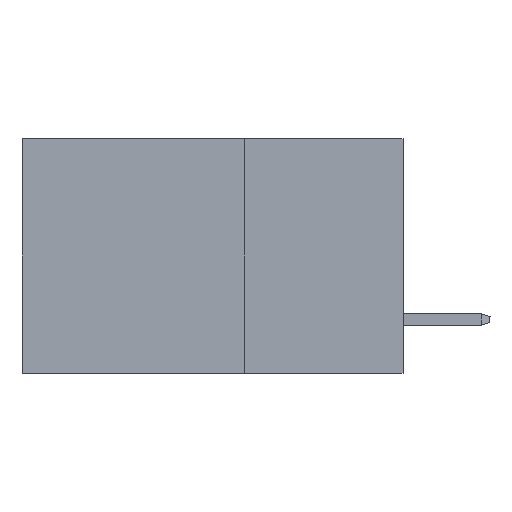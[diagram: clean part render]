
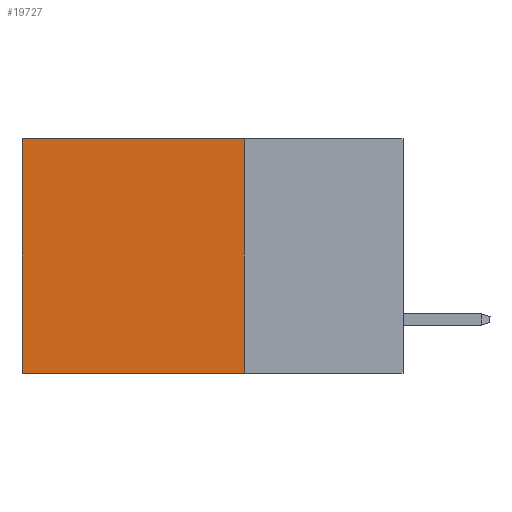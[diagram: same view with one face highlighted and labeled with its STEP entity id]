
A CAD part, left-side view. The second image highlights one B-rep face of the part: STEP entity #19727.
In plain terms, the highlighted planar face has unit normal (-1, 0, 0).
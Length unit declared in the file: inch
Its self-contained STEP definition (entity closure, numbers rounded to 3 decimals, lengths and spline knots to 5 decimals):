
#1420 = AXIS2_PLACEMENT_3D ( 'NONE', #20679, #16460, #16831 ) ;
#1966 = LINE ( 'NONE', #21075, #5187 ) ;
#2099 = ORIENTED_EDGE ( 'NONE', *, *, #12892, .T. ) ;
#4251 = EDGE_CURVE ( 'NONE', #16818, #9234, #8527, .T. ) ;
#4385 = ORIENTED_EDGE ( 'NONE', *, *, #4251, .F. ) ;
#4425 = CARTESIAN_POINT ( 'NONE',  ( 0.2875, 0.6, -0.37 ) ) ;
#4643 = CARTESIAN_POINT ( 'NONE',  ( 0.2875, 0.6, 0. ) ) ;
#5187 = VECTOR ( 'NONE', #5882, 39.37008 ) ;
#5875 = CARTESIAN_POINT ( 'NONE',  ( 0.2875, 0.25, -0.37 ) ) ;
#5882 = DIRECTION ( 'NONE',  ( 0., 1., 0. ) ) ;
#6618 = DIRECTION ( 'NONE',  ( 0., 0., -1. ) ) ;
#8527 = LINE ( 'NONE', #12297, #21005 ) ;
#8618 = EDGE_CURVE ( 'NONE', #22984, #16818, #14088, .T. ) ;
#8728 = FACE_OUTER_BOUND ( 'NONE', #24660, .T. ) ;
#9094 = VERTEX_POINT ( 'NONE', #15432 ) ;
#9234 = VERTEX_POINT ( 'NONE', #4425 ) ;
#10209 = ORIENTED_EDGE ( 'NONE', *, *, #8618, .F. ) ;
#10867 = ORIENTED_EDGE ( 'NONE', *, *, #24221, .T. ) ;
#12297 = CARTESIAN_POINT ( 'NONE',  ( 0.2875, 0.25, -0.37 ) ) ;
#12305 = DIRECTION ( 'NONE',  ( 0., 0., -1. ) ) ;
#12556 = DIRECTION ( 'NONE',  ( 0., 1., 0. ) ) ;
#12892 = EDGE_CURVE ( 'NONE', #22984, #9094, #1966, .T. ) ;
#14088 = LINE ( 'NONE', #21705, #23809 ) ;
#14683 = PLANE ( 'NONE',  #1420 ) ;
#15250 = VECTOR ( 'NONE', #12305, 39.37008 ) ;
#15432 = CARTESIAN_POINT ( 'NONE',  ( 0.2875, 0.6, 0. ) ) ;
#16121 = LINE ( 'NONE', #4643, #15250 ) ;
#16460 = DIRECTION ( 'NONE',  ( 1., 0., 0. ) ) ;
#16818 = VERTEX_POINT ( 'NONE', #5875 ) ;
#16831 = DIRECTION ( 'NONE',  ( 0., 0., -1. ) ) ;
#19727 = ADVANCED_FACE ( 'NONE', ( #8728 ), #14683, .F. ) ;
#20679 = CARTESIAN_POINT ( 'NONE',  ( 0.2875, 0.25, 0. ) ) ;
#21005 = VECTOR ( 'NONE', #12556, 39.37008 ) ;
#21075 = CARTESIAN_POINT ( 'NONE',  ( 0.2875, 0.25, 0. ) ) ;
#21705 = CARTESIAN_POINT ( 'NONE',  ( 0.2875, 0.25, 0. ) ) ;
#22091 = CARTESIAN_POINT ( 'NONE',  ( 0.2875, 0.25, 0. ) ) ;
#22984 = VERTEX_POINT ( 'NONE', #22091 ) ;
#23809 = VECTOR ( 'NONE', #6618, 39.37008 ) ;
#24221 = EDGE_CURVE ( 'NONE', #9094, #9234, #16121, .T. ) ;
#24660 = EDGE_LOOP ( 'NONE', ( #10867, #4385, #10209, #2099 ) ) ;
